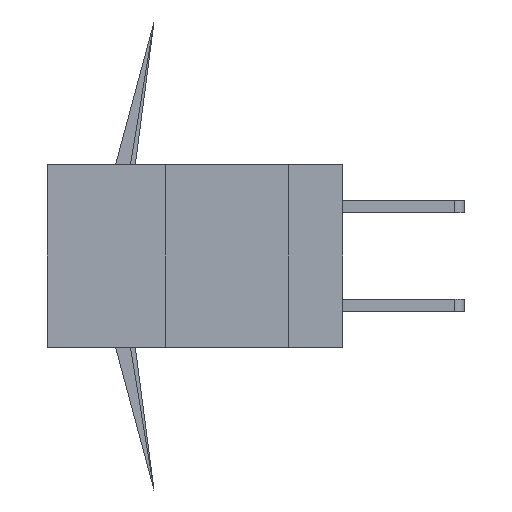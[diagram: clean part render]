
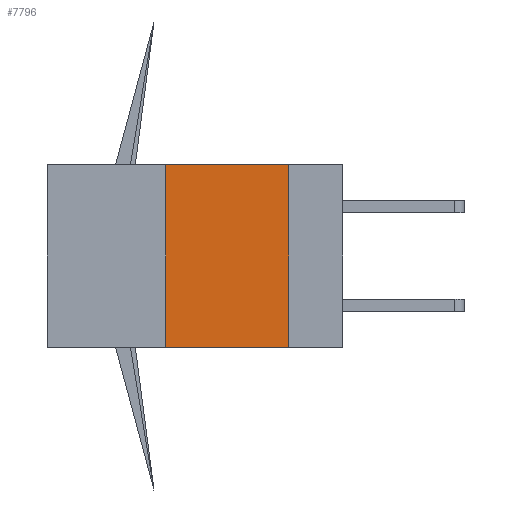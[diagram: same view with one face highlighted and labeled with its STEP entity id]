
A CAD part, left-side view. The second image highlights one B-rep face of the part: STEP entity #7796.
In plain terms, the highlighted planar face has unit normal (-1, 0, 0).
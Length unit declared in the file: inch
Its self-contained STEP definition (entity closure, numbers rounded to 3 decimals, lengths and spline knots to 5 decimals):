
#42 = EDGE_LOOP ( 'NONE', ( #1796, #4404, #6851, #9177 ) ) ;
#361 = VECTOR ( 'NONE', #10419, 39.37008 ) ;
#1281 = VERTEX_POINT ( 'NONE', #4737 ) ;
#1624 = LINE ( 'NONE', #2614, #10393 ) ;
#1796 = ORIENTED_EDGE ( 'NONE', *, *, #4902, .F. ) ;
#1987 = VERTEX_POINT ( 'NONE', #9932 ) ;
#2614 = CARTESIAN_POINT ( 'NONE',  ( 0., 0.6, -0.37 ) ) ;
#2939 = LINE ( 'NONE', #6140, #361 ) ;
#2982 = PLANE ( 'NONE',  #10515 ) ;
#3508 = VERTEX_POINT ( 'NONE', #5042 ) ;
#3850 = CARTESIAN_POINT ( 'NONE',  ( 0., 0.11, -0.37 ) ) ;
#3864 = VECTOR ( 'NONE', #9470, 39.37008 ) ;
#4030 = DIRECTION ( 'NONE',  ( 1., 0., 0. ) ) ;
#4273 = DIRECTION ( 'NONE',  ( 0., 0., -1. ) ) ;
#4404 = ORIENTED_EDGE ( 'NONE', *, *, #7005, .F. ) ;
#4737 = CARTESIAN_POINT ( 'NONE',  ( 0., 0.36, 0. ) ) ;
#4902 = EDGE_CURVE ( 'NONE', #3508, #9543, #10624, .T. ) ;
#5042 = CARTESIAN_POINT ( 'NONE',  ( 0., 0.11, 0. ) ) ;
#5639 = FACE_OUTER_BOUND ( 'NONE', #42, .T. ) ;
#6081 = VECTOR ( 'NONE', #4273, 39.37008 ) ;
#6140 = CARTESIAN_POINT ( 'NONE',  ( 0., 0.36, 0. ) ) ;
#6851 = ORIENTED_EDGE ( 'NONE', *, *, #11459, .F. ) ;
#7005 = EDGE_CURVE ( 'NONE', #1281, #3508, #10581, .T. ) ;
#7796 = ADVANCED_FACE ( 'NONE', ( #5639 ), #2982, .F. ) ;
#7954 = CARTESIAN_POINT ( 'NONE',  ( 0., 0.11, 0. ) ) ;
#8537 = CARTESIAN_POINT ( 'NONE',  ( 0., 0.6, 0. ) ) ;
#8683 = CARTESIAN_POINT ( 'NONE',  ( 0., 0.6, 0. ) ) ;
#9177 = ORIENTED_EDGE ( 'NONE', *, *, #10966, .T. ) ;
#9470 = DIRECTION ( 'NONE',  ( 0., -1., 0. ) ) ;
#9543 = VERTEX_POINT ( 'NONE', #3850 ) ;
#9932 = CARTESIAN_POINT ( 'NONE',  ( 0., 0.36, -0.37 ) ) ;
#10202 = DIRECTION ( 'NONE',  ( 0., 0., -1. ) ) ;
#10393 = VECTOR ( 'NONE', #10666, 39.37008 ) ;
#10419 = DIRECTION ( 'NONE',  ( 0., 0., 1. ) ) ;
#10515 = AXIS2_PLACEMENT_3D ( 'NONE', #8537, #4030, #10202 ) ;
#10581 = LINE ( 'NONE', #8683, #3864 ) ;
#10624 = LINE ( 'NONE', #7954, #6081 ) ;
#10666 = DIRECTION ( 'NONE',  ( 0., -1., 0. ) ) ;
#10966 = EDGE_CURVE ( 'NONE', #1987, #9543, #1624, .T. ) ;
#11459 = EDGE_CURVE ( 'NONE', #1987, #1281, #2939, .T. ) ;
